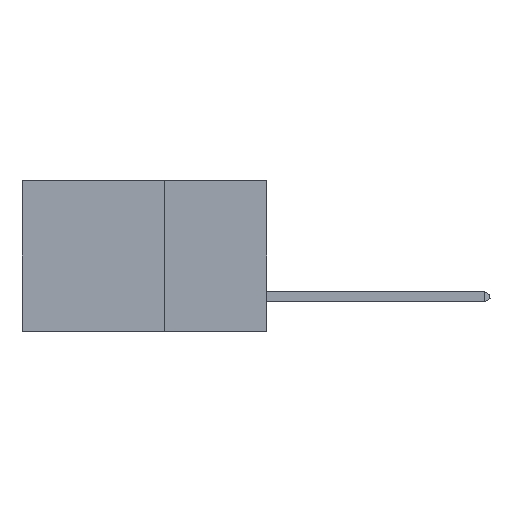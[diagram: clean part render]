
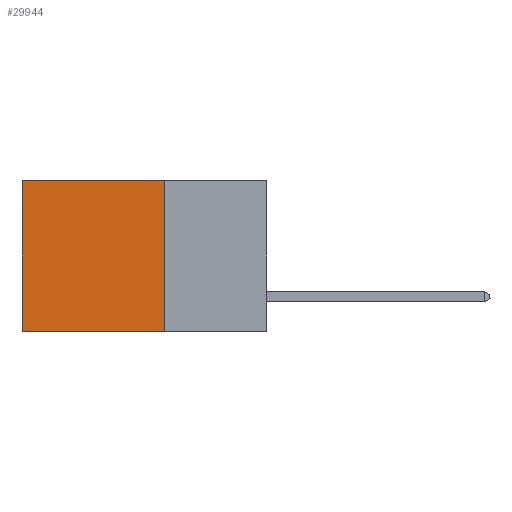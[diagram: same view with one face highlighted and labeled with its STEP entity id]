
A CAD part, left-side view. The second image highlights one B-rep face of the part: STEP entity #29944.
In plain terms, the highlighted planar face has unit normal (-1, 0, 0).
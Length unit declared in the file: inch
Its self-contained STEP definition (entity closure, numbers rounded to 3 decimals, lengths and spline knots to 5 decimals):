
#766 = VECTOR ( 'NONE', #29416, 39.37008 ) ;
#4557 = DIRECTION ( 'NONE',  ( 0., 0., -1. ) ) ;
#4879 = EDGE_CURVE ( 'NONE', #23353, #12444, #9010, .T. ) ;
#5124 = ORIENTED_EDGE ( 'NONE', *, *, #25600, .T. ) ;
#7073 = DIRECTION ( 'NONE',  ( 0., 1., 0. ) ) ;
#8997 = VERTEX_POINT ( 'NONE', #11251 ) ;
#9010 = LINE ( 'NONE', #20240, #766 ) ;
#11251 = CARTESIAN_POINT ( 'NONE',  ( 0.2875, 0.6, -0.37 ) ) ;
#12444 = VERTEX_POINT ( 'NONE', #26964 ) ;
#12894 = VECTOR ( 'NONE', #4557, 39.37008 ) ;
#13659 = LINE ( 'NONE', #34966, #38000 ) ;
#13802 = DIRECTION ( 'NONE',  ( 1., 0., 0. ) ) ;
#16291 = VECTOR ( 'NONE', #7073, 39.37008 ) ;
#16779 = DIRECTION ( 'NONE',  ( 0., 1., 0. ) ) ;
#18005 = CARTESIAN_POINT ( 'NONE',  ( 0.2875, 0.25, 0. ) ) ;
#18260 = ORIENTED_EDGE ( 'NONE', *, *, #19624, .T. ) ;
#19256 = CARTESIAN_POINT ( 'NONE',  ( 0.2875, 0.25, 0. ) ) ;
#19624 = EDGE_CURVE ( 'NONE', #25480, #8997, #37213, .T. ) ;
#20240 = CARTESIAN_POINT ( 'NONE',  ( 0.2875, 0.25, 0. ) ) ;
#21758 = EDGE_CURVE ( 'NONE', #12444, #8997, #13659, .T. ) ;
#21791 = ORIENTED_EDGE ( 'NONE', *, *, #21758, .F. ) ;
#23353 = VERTEX_POINT ( 'NONE', #18005 ) ;
#25480 = VERTEX_POINT ( 'NONE', #33860 ) ;
#25600 = EDGE_CURVE ( 'NONE', #23353, #25480, #32446, .T. ) ;
#26007 = CARTESIAN_POINT ( 'NONE',  ( 0.2875, 0.25, 0. ) ) ;
#26964 = CARTESIAN_POINT ( 'NONE',  ( 0.2875, 0.25, -0.37 ) ) ;
#27064 = AXIS2_PLACEMENT_3D ( 'NONE', #26007, #13802, #35110 ) ;
#29383 = ORIENTED_EDGE ( 'NONE', *, *, #4879, .F. ) ;
#29416 = DIRECTION ( 'NONE',  ( 0., 0., -1. ) ) ;
#29944 = ADVANCED_FACE ( 'NONE', ( #38078 ), #32045, .F. ) ;
#32045 = PLANE ( 'NONE',  #27064 ) ;
#32446 = LINE ( 'NONE', #19256, #16291 ) ;
#33860 = CARTESIAN_POINT ( 'NONE',  ( 0.2875, 0.6, 0. ) ) ;
#34205 = EDGE_LOOP ( 'NONE', ( #18260, #21791, #29383, #5124 ) ) ;
#34966 = CARTESIAN_POINT ( 'NONE',  ( 0.2875, 0.25, -0.37 ) ) ;
#34982 = CARTESIAN_POINT ( 'NONE',  ( 0.2875, 0.6, 0. ) ) ;
#35110 = DIRECTION ( 'NONE',  ( 0., 0., -1. ) ) ;
#37213 = LINE ( 'NONE', #34982, #12894 ) ;
#38000 = VECTOR ( 'NONE', #16779, 39.37008 ) ;
#38078 = FACE_OUTER_BOUND ( 'NONE', #34205, .T. ) ;
